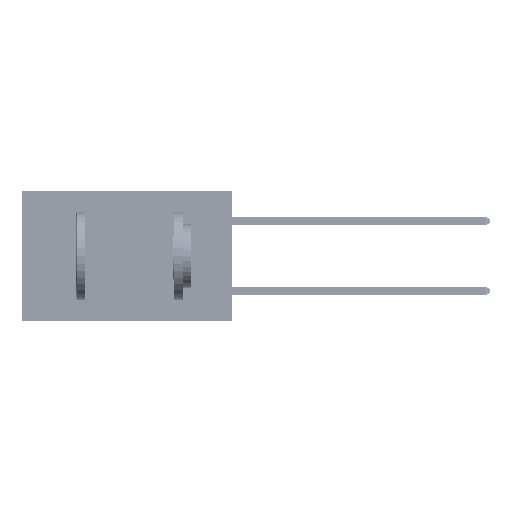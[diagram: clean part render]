
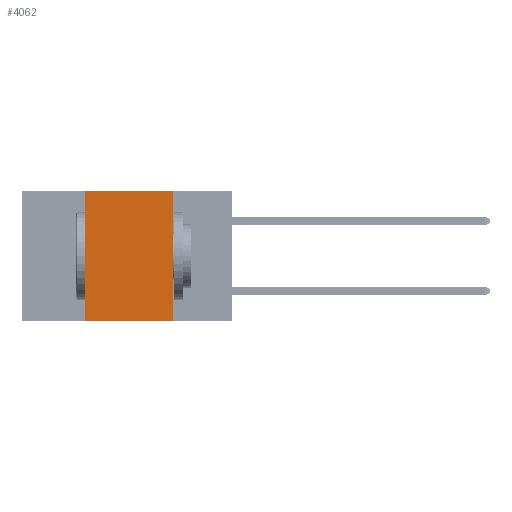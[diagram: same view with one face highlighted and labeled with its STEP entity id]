
A CAD part, left-side view. The second image highlights one B-rep face of the part: STEP entity #4062.
In plain terms, the highlighted planar face has unit normal (-1, 0, 0).
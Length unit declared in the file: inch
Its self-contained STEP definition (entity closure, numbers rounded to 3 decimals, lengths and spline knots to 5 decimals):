
#1445 = AXIS2_PLACEMENT_3D ( 'NONE', #3004, #36097, #25130 ) ;
#1725 = VECTOR ( 'NONE', #31969, 39.37008 ) ;
#2027 = VECTOR ( 'NONE', #21764, 39.37008 ) ;
#2699 = LINE ( 'NONE', #33769, #2027 ) ;
#2949 = DIRECTION ( 'NONE',  ( 0., -1., 0. ) ) ;
#3004 = CARTESIAN_POINT ( 'NONE',  ( 0., 0.6, 0. ) ) ;
#4062 = ADVANCED_FACE ( 'NONE', ( #22108 ), #23728, .F. ) ;
#9595 = VERTEX_POINT ( 'NONE', #51095 ) ;
#9843 = ORIENTED_EDGE ( 'NONE', *, *, #41461, .F. ) ;
#10851 = CARTESIAN_POINT ( 'NONE',  ( 0., 0.6, 0. ) ) ;
#13064 = ORIENTED_EDGE ( 'NONE', *, *, #24283, .F. ) ;
#20961 = LINE ( 'NONE', #10851, #25428 ) ;
#21764 = DIRECTION ( 'NONE',  ( 0., -1., 0. ) ) ;
#22108 = FACE_OUTER_BOUND ( 'NONE', #41742, .T. ) ;
#23728 = PLANE ( 'NONE',  #1445 ) ;
#24251 = VERTEX_POINT ( 'NONE', #36105 ) ;
#24283 = EDGE_CURVE ( 'NONE', #9595, #24251, #37465, .T. ) ;
#24582 = DIRECTION ( 'NONE',  ( 0., 0., -1. ) ) ;
#24925 = LINE ( 'NONE', #32340, #1725 ) ;
#25130 = DIRECTION ( 'NONE',  ( 0., 0., -1. ) ) ;
#25428 = VECTOR ( 'NONE', #2949, 39.37008 ) ;
#28072 = CARTESIAN_POINT ( 'NONE',  ( 0., 0.42, 0. ) ) ;
#28209 = CARTESIAN_POINT ( 'NONE',  ( 0., 0.17, 0. ) ) ;
#31969 = DIRECTION ( 'NONE',  ( 0., 0., 1. ) ) ;
#32340 = CARTESIAN_POINT ( 'NONE',  ( 0., 0.42, 0. ) ) ;
#33769 = CARTESIAN_POINT ( 'NONE',  ( 0., 0.6, -0.37 ) ) ;
#34622 = EDGE_CURVE ( 'NONE', #37000, #9595, #20961, .T. ) ;
#35664 = EDGE_CURVE ( 'NONE', #38248, #24251, #2699, .T. ) ;
#36097 = DIRECTION ( 'NONE',  ( 1., 0., 0. ) ) ;
#36105 = CARTESIAN_POINT ( 'NONE',  ( 0., 0.17, -0.37 ) ) ;
#36902 = CARTESIAN_POINT ( 'NONE',  ( 0., 0.42, -0.37 ) ) ;
#37000 = VERTEX_POINT ( 'NONE', #28072 ) ;
#37465 = LINE ( 'NONE', #28209, #42624 ) ;
#38248 = VERTEX_POINT ( 'NONE', #36902 ) ;
#38998 = ORIENTED_EDGE ( 'NONE', *, *, #34622, .F. ) ;
#41461 = EDGE_CURVE ( 'NONE', #38248, #37000, #24925, .T. ) ;
#41742 = EDGE_LOOP ( 'NONE', ( #13064, #38998, #9843, #41887 ) ) ;
#41887 = ORIENTED_EDGE ( 'NONE', *, *, #35664, .T. ) ;
#42624 = VECTOR ( 'NONE', #24582, 39.37008 ) ;
#51095 = CARTESIAN_POINT ( 'NONE',  ( 0., 0.17, 0. ) ) ;
